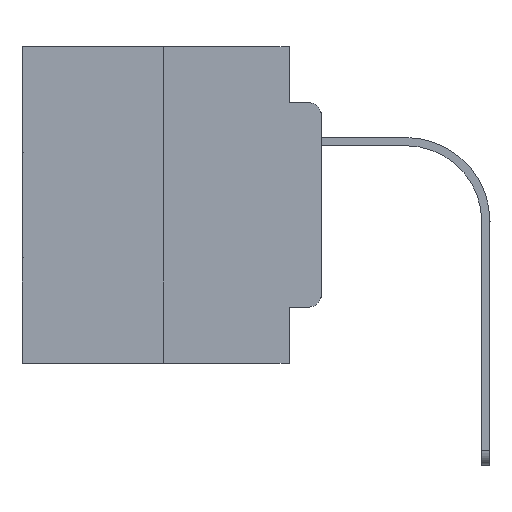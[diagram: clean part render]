
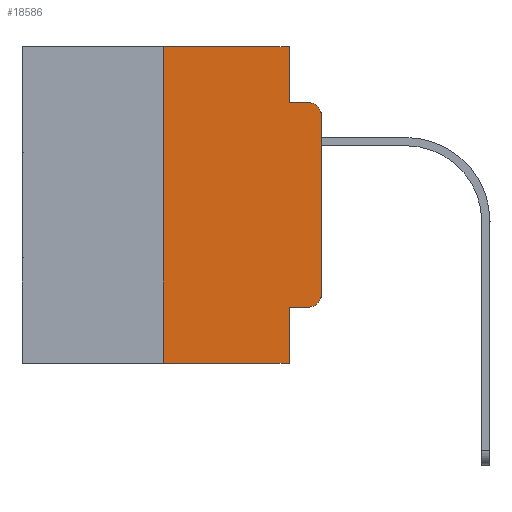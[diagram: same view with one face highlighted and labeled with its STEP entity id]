
A CAD part, left-side view. The second image highlights one B-rep face of the part: STEP entity #18586.
In plain terms, the highlighted planar face has unit normal (-1, 0, 0).
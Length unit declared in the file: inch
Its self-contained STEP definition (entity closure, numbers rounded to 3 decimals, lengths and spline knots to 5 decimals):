
#419 = EDGE_CURVE ( 'NONE', #6747, #23363, #11571, .T. ) ;
#447 = CARTESIAN_POINT ( 'NONE',  ( 0., 0.25, -0.5 ) ) ;
#1057 = DIRECTION ( 'NONE',  ( 0., -1., 0. ) ) ;
#1136 = CIRCLE ( 'NONE', #17237, 0.02 ) ;
#1278 = CARTESIAN_POINT ( 'NONE',  ( 0., 0.473, -0.5 ) ) ;
#1290 = CARTESIAN_POINT ( 'NONE',  ( 0., 0.051, -0.4115 ) ) ;
#1345 = EDGE_CURVE ( 'NONE', #17921, #2587, #3683, .T. ) ;
#1684 = LINE ( 'NONE', #19227, #4291 ) ;
#2587 = VERTEX_POINT ( 'NONE', #15694 ) ;
#2784 = VERTEX_POINT ( 'NONE', #5760 ) ;
#3683 = LINE ( 'NONE', #7859, #28196 ) ;
#3914 = EDGE_CURVE ( 'NONE', #16093, #2784, #12965, .T. ) ;
#4139 = EDGE_CURVE ( 'NONE', #17921, #18033, #25303, .T. ) ;
#4291 = VECTOR ( 'NONE', #24232, 39.37008 ) ;
#5079 = PLANE ( 'NONE',  #23051 ) ;
#5080 = VECTOR ( 'NONE', #23135, 39.37008 ) ;
#5553 = EDGE_CURVE ( 'NONE', #23363, #16093, #8677, .T. ) ;
#5760 = CARTESIAN_POINT ( 'NONE',  ( 0., 0., -0.1085 ) ) ;
#6455 = ORIENTED_EDGE ( 'NONE', *, *, #21468, .F. ) ;
#6747 = VERTEX_POINT ( 'NONE', #1290 ) ;
#6894 = VECTOR ( 'NONE', #23443, 39.37008 ) ;
#7859 = CARTESIAN_POINT ( 'NONE',  ( 0., 0.25, 0. ) ) ;
#7958 = LINE ( 'NONE', #10134, #27674 ) ;
#8050 = VECTOR ( 'NONE', #9123, 39.37008 ) ;
#8677 = CIRCLE ( 'NONE', #17856, 0.02 ) ;
#8856 = ORIENTED_EDGE ( 'NONE', *, *, #419, .T. ) ;
#9106 = EDGE_CURVE ( 'NONE', #2784, #20762, #1136, .T. ) ;
#9123 = DIRECTION ( 'NONE',  ( 0., -1., 0. ) ) ;
#9547 = CARTESIAN_POINT ( 'NONE',  ( 0., 0.051, 0. ) ) ;
#10134 = CARTESIAN_POINT ( 'NONE',  ( 0., 0.051, -0.0885 ) ) ;
#10687 = DIRECTION ( 'NONE',  ( 0., 0., -1. ) ) ;
#11302 = VERTEX_POINT ( 'NONE', #12567 ) ;
#11571 = LINE ( 'NONE', #15482, #8050 ) ;
#11723 = CARTESIAN_POINT ( 'NONE',  ( 0., 0.473, 0. ) ) ;
#12464 = CARTESIAN_POINT ( 'NONE',  ( 0., 0., -0.3915 ) ) ;
#12518 = DIRECTION ( 'NONE',  ( 0., 0., -1. ) ) ;
#12567 = CARTESIAN_POINT ( 'NONE',  ( 0., 0.051, 0. ) ) ;
#12583 = EDGE_LOOP ( 'NONE', ( #13982, #23498, #24308, #6455, #13026, #17821, #13657, #14183, #8856, #15736 ) ) ;
#12806 = CARTESIAN_POINT ( 'NONE',  ( 0., 0.051, 0. ) ) ;
#12965 = LINE ( 'NONE', #23727, #6894 ) ;
#13026 = ORIENTED_EDGE ( 'NONE', *, *, #23097, .F. ) ;
#13657 = ORIENTED_EDGE ( 'NONE', *, *, #4139, .T. ) ;
#13733 = EDGE_CURVE ( 'NONE', #20282, #20762, #7958, .T. ) ;
#13874 = DIRECTION ( 'NONE',  ( 1., 0., 0. ) ) ;
#13982 = ORIENTED_EDGE ( 'NONE', *, *, #3914, .T. ) ;
#14183 = ORIENTED_EDGE ( 'NONE', *, *, #15239, .F. ) ;
#14300 = DIRECTION ( 'NONE',  ( 0., 0., -1. ) ) ;
#14688 = CARTESIAN_POINT ( 'NONE',  ( 0., 0.02, -0.3915 ) ) ;
#15105 = CARTESIAN_POINT ( 'NONE',  ( 0., 0.051, -0.0885 ) ) ;
#15239 = EDGE_CURVE ( 'NONE', #6747, #18033, #23192, .T. ) ;
#15482 = CARTESIAN_POINT ( 'NONE',  ( 0., 0.051, -0.4115 ) ) ;
#15694 = CARTESIAN_POINT ( 'NONE',  ( 0., 0.25, 0. ) ) ;
#15736 = ORIENTED_EDGE ( 'NONE', *, *, #5553, .T. ) ;
#16093 = VERTEX_POINT ( 'NONE', #12464 ) ;
#16694 = LINE ( 'NONE', #12806, #24361 ) ;
#17237 = AXIS2_PLACEMENT_3D ( 'NONE', #22019, #28235, #17313 ) ;
#17313 = DIRECTION ( 'NONE',  ( 0., 0., -1. ) ) ;
#17821 = ORIENTED_EDGE ( 'NONE', *, *, #1345, .F. ) ;
#17856 = AXIS2_PLACEMENT_3D ( 'NONE', #14688, #19262, #12518 ) ;
#17921 = VERTEX_POINT ( 'NONE', #447 ) ;
#18033 = VERTEX_POINT ( 'NONE', #20165 ) ;
#18586 = ADVANCED_FACE ( 'NONE', ( #26963 ), #5079, .F. ) ;
#19227 = CARTESIAN_POINT ( 'NONE',  ( 0., 0.473, 0. ) ) ;
#19262 = DIRECTION ( 'NONE',  ( -1., 0., 0. ) ) ;
#20165 = CARTESIAN_POINT ( 'NONE',  ( 0., 0.051, -0.5 ) ) ;
#20282 = VERTEX_POINT ( 'NONE', #15105 ) ;
#20762 = VERTEX_POINT ( 'NONE', #22029 ) ;
#21468 = EDGE_CURVE ( 'NONE', #11302, #20282, #16694, .T. ) ;
#22019 = CARTESIAN_POINT ( 'NONE',  ( 0., 0.02, -0.1085 ) ) ;
#22029 = CARTESIAN_POINT ( 'NONE',  ( 0., 0.02, -0.0885 ) ) ;
#23051 = AXIS2_PLACEMENT_3D ( 'NONE', #11723, #13874, #10687 ) ;
#23097 = EDGE_CURVE ( 'NONE', #2587, #11302, #1684, .T. ) ;
#23135 = DIRECTION ( 'NONE',  ( 0., -1., 0. ) ) ;
#23192 = LINE ( 'NONE', #9547, #27154 ) ;
#23363 = VERTEX_POINT ( 'NONE', #23533 ) ;
#23443 = DIRECTION ( 'NONE',  ( 0., 0., 1. ) ) ;
#23498 = ORIENTED_EDGE ( 'NONE', *, *, #9106, .T. ) ;
#23533 = CARTESIAN_POINT ( 'NONE',  ( 0., 0.02, -0.4115 ) ) ;
#23727 = CARTESIAN_POINT ( 'NONE',  ( 0., 0., 0. ) ) ;
#24232 = DIRECTION ( 'NONE',  ( 0., -1., 0. ) ) ;
#24308 = ORIENTED_EDGE ( 'NONE', *, *, #13733, .F. ) ;
#24361 = VECTOR ( 'NONE', #28041, 39.37008 ) ;
#25303 = LINE ( 'NONE', #1278, #5080 ) ;
#26963 = FACE_OUTER_BOUND ( 'NONE', #12583, .T. ) ;
#27154 = VECTOR ( 'NONE', #14300, 39.37008 ) ;
#27674 = VECTOR ( 'NONE', #1057, 39.37008 ) ;
#27719 = DIRECTION ( 'NONE',  ( 0., 0., 1. ) ) ;
#28041 = DIRECTION ( 'NONE',  ( 0., 0., -1. ) ) ;
#28196 = VECTOR ( 'NONE', #27719, 39.37008 ) ;
#28235 = DIRECTION ( 'NONE',  ( -1., 0., 0. ) ) ;
